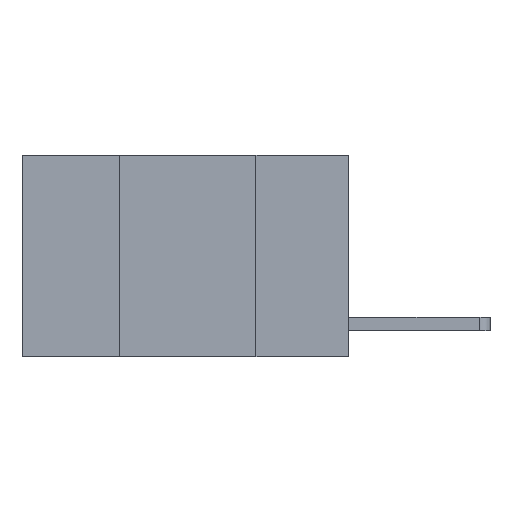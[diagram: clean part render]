
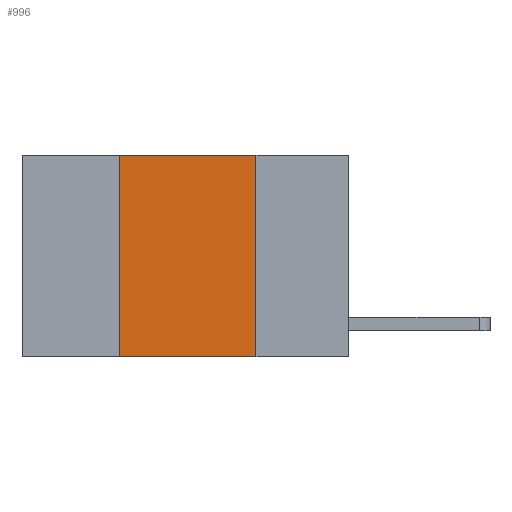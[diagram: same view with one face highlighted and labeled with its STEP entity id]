
A CAD part, left-side view. The second image highlights one B-rep face of the part: STEP entity #996.
In plain terms, the highlighted planar face has unit normal (-1, 0, 0).
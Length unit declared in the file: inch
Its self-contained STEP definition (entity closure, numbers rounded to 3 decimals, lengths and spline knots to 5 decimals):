
#523 = VERTEX_POINT ( 'NONE', #1071 ) ;
#541 = VECTOR ( 'NONE', #4273, 39.37008 ) ;
#996 = ADVANCED_FACE ( 'NONE', ( #5840 ), #1432, .F. ) ;
#1071 = CARTESIAN_POINT ( 'NONE',  ( 0., 0.42, -0.37 ) ) ;
#1137 = CARTESIAN_POINT ( 'NONE',  ( 0., 0.42, 0. ) ) ;
#1189 = EDGE_CURVE ( 'NONE', #3364, #9163, #4017, .T. ) ;
#1432 = PLANE ( 'NONE',  #8483 ) ;
#1844 = VECTOR ( 'NONE', #9307, 39.37008 ) ;
#2513 = LINE ( 'NONE', #7322, #541 ) ;
#2603 = ORIENTED_EDGE ( 'NONE', *, *, #5874, .T. ) ;
#3112 = CARTESIAN_POINT ( 'NONE',  ( 0., 0.17, -0.37 ) ) ;
#3304 = ORIENTED_EDGE ( 'NONE', *, *, #6511, .F. ) ;
#3316 = ORIENTED_EDGE ( 'NONE', *, *, #8080, .F. ) ;
#3340 = CARTESIAN_POINT ( 'NONE',  ( 0., 0.17, 0. ) ) ;
#3364 = VERTEX_POINT ( 'NONE', #3340 ) ;
#3607 = VECTOR ( 'NONE', #7520, 39.37008 ) ;
#3818 = EDGE_LOOP ( 'NONE', ( #5510, #3316, #3304, #2603 ) ) ;
#3840 = LINE ( 'NONE', #8650, #1844 ) ;
#4017 = LINE ( 'NONE', #5302, #3607 ) ;
#4273 = DIRECTION ( 'NONE',  ( 0., -1., 0. ) ) ;
#4429 = DIRECTION ( 'NONE',  ( 0., 0., -1. ) ) ;
#4573 = CARTESIAN_POINT ( 'NONE',  ( 0., 0.6, 0. ) ) ;
#5302 = CARTESIAN_POINT ( 'NONE',  ( 0., 0.17, 0. ) ) ;
#5510 = ORIENTED_EDGE ( 'NONE', *, *, #1189, .F. ) ;
#5780 = DIRECTION ( 'NONE',  ( 0., 0., 1. ) ) ;
#5840 = FACE_OUTER_BOUND ( 'NONE', #3818, .T. ) ;
#5874 = EDGE_CURVE ( 'NONE', #523, #9163, #3840, .T. ) ;
#6511 = EDGE_CURVE ( 'NONE', #523, #7640, #8640, .T. ) ;
#6751 = VECTOR ( 'NONE', #5780, 39.37008 ) ;
#6889 = CARTESIAN_POINT ( 'NONE',  ( 0., 0.42, 0. ) ) ;
#7322 = CARTESIAN_POINT ( 'NONE',  ( 0., 0.6, 0. ) ) ;
#7520 = DIRECTION ( 'NONE',  ( 0., 0., -1. ) ) ;
#7640 = VERTEX_POINT ( 'NONE', #6889 ) ;
#7741 = DIRECTION ( 'NONE',  ( 1., 0., 0. ) ) ;
#8080 = EDGE_CURVE ( 'NONE', #7640, #3364, #2513, .T. ) ;
#8483 = AXIS2_PLACEMENT_3D ( 'NONE', #4573, #7741, #4429 ) ;
#8640 = LINE ( 'NONE', #1137, #6751 ) ;
#8650 = CARTESIAN_POINT ( 'NONE',  ( 0., 0.6, -0.37 ) ) ;
#9163 = VERTEX_POINT ( 'NONE', #3112 ) ;
#9307 = DIRECTION ( 'NONE',  ( 0., -1., 0. ) ) ;
